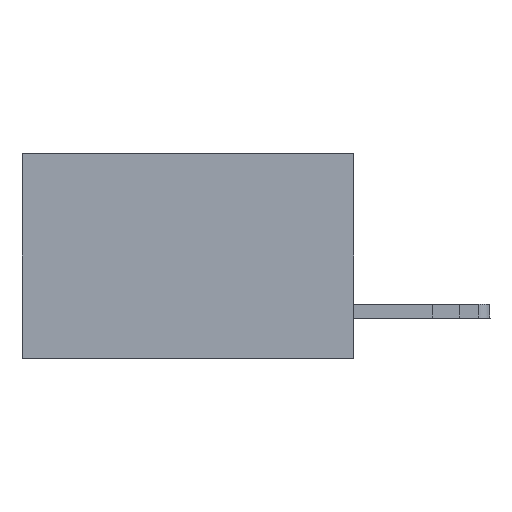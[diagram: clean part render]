
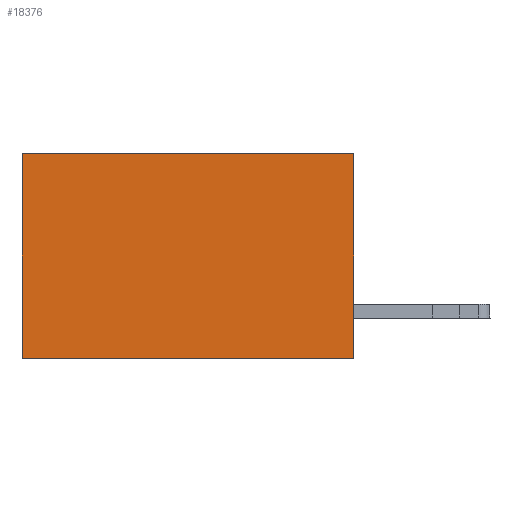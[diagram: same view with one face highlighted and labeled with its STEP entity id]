
A CAD part, left-side view. The second image highlights one B-rep face of the part: STEP entity #18376.
In plain terms, the highlighted planar face has unit normal (-1, 0, 0).
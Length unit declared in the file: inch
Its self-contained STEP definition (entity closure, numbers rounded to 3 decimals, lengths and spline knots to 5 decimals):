
#66 = VECTOR ( 'NONE', #6412, 39.37008 ) ;
#1027 = PLANE ( 'NONE',  #17976 ) ;
#1402 = CARTESIAN_POINT ( 'NONE',  ( 0.2875, 0., 0. ) ) ;
#1433 = ORIENTED_EDGE ( 'NONE', *, *, #3868, .T. ) ;
#1877 = VECTOR ( 'NONE', #10311, 39.37008 ) ;
#2079 = EDGE_CURVE ( 'NONE', #8355, #12012, #4437, .T. ) ;
#2434 = CARTESIAN_POINT ( 'NONE',  ( 0.2875, 0., -0.37 ) ) ;
#3868 = EDGE_CURVE ( 'NONE', #9824, #4196, #6716, .T. ) ;
#4196 = VERTEX_POINT ( 'NONE', #9118 ) ;
#4437 = LINE ( 'NONE', #4704, #66 ) ;
#4704 = CARTESIAN_POINT ( 'NONE',  ( 0.2875, 0., 0. ) ) ;
#4808 = LINE ( 'NONE', #2434, #16581 ) ;
#6130 = EDGE_CURVE ( 'NONE', #12012, #4196, #4808, .T. ) ;
#6412 = DIRECTION ( 'NONE',  ( 0., 0., -1. ) ) ;
#6716 = LINE ( 'NONE', #16630, #1877 ) ;
#7605 = DIRECTION ( 'NONE',  ( 1., 0., 0. ) ) ;
#8355 = VERTEX_POINT ( 'NONE', #18831 ) ;
#9034 = DIRECTION ( 'NONE',  ( 0., 1., 0. ) ) ;
#9118 = CARTESIAN_POINT ( 'NONE',  ( 0.2875, 0.6, -0.37 ) ) ;
#9824 = VERTEX_POINT ( 'NONE', #18995 ) ;
#10311 = DIRECTION ( 'NONE',  ( 0., 0., -1. ) ) ;
#10579 = CARTESIAN_POINT ( 'NONE',  ( 0.2875, 0., -0.37 ) ) ;
#10869 = ORIENTED_EDGE ( 'NONE', *, *, #2079, .F. ) ;
#12012 = VERTEX_POINT ( 'NONE', #10579 ) ;
#13953 = ORIENTED_EDGE ( 'NONE', *, *, #18502, .T. ) ;
#15230 = FACE_OUTER_BOUND ( 'NONE', #20428, .T. ) ;
#15858 = DIRECTION ( 'NONE',  ( 0., 1., 0. ) ) ;
#16434 = VECTOR ( 'NONE', #15858, 39.37008 ) ;
#16581 = VECTOR ( 'NONE', #9034, 39.37008 ) ;
#16630 = CARTESIAN_POINT ( 'NONE',  ( 0.2875, 0.6, 0. ) ) ;
#17976 = AXIS2_PLACEMENT_3D ( 'NONE', #20130, #7605, #18622 ) ;
#18376 = ADVANCED_FACE ( 'NONE', ( #15230 ), #1027, .F. ) ;
#18502 = EDGE_CURVE ( 'NONE', #8355, #9824, #20563, .T. ) ;
#18622 = DIRECTION ( 'NONE',  ( 0., 0., -1. ) ) ;
#18831 = CARTESIAN_POINT ( 'NONE',  ( 0.2875, 0., 0. ) ) ;
#18995 = CARTESIAN_POINT ( 'NONE',  ( 0.2875, 0.6, 0. ) ) ;
#19196 = ORIENTED_EDGE ( 'NONE', *, *, #6130, .F. ) ;
#20130 = CARTESIAN_POINT ( 'NONE',  ( 0.2875, 0., 0. ) ) ;
#20428 = EDGE_LOOP ( 'NONE', ( #1433, #19196, #10869, #13953 ) ) ;
#20563 = LINE ( 'NONE', #1402, #16434 ) ;
